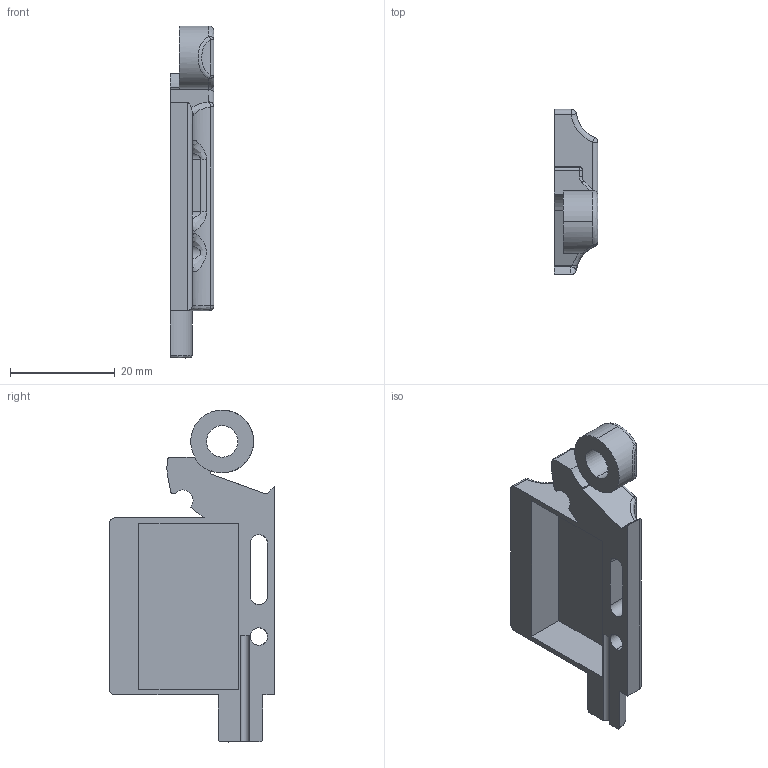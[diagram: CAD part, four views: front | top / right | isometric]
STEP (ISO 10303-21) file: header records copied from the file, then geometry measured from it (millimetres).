
FILE_DESCRIPTION (( 'STEP AP214' ), '1' );
FILE_NAME ('Imura_V3_Striker_Right.step', '2015-04-30T21:15:10', ( 'WarFairy' ), ( '' ), 'SwSTEP 2.0', 'SolidWorks 2013', '' );
FILE_SCHEMA (( 'AUTOMOTIVE_DESIGN' ));
Length unit declared in the file: millimetre
Products named in the file (1): Imura_V3_Striker_Right
Bounding box: 8.35 x 31.5 x 63.35 mm (x, y, z)
Volume: 4736.6 mm3; surface area: 4932.9 mm2
Topology: 1 solids, 1 shells, 107 faces, 271 edges, 159 vertices
Faces by surface type: cylinder 45, bspline 33, plane 25, torus 3, sphere 1
Entity records: 4877 total; most frequent: CARTESIAN_POINT 2529, ORIENTED_EDGE 530, DIRECTION 434, EDGE_CURVE 265, AXIS2_PLACEMENT_3D 161, VERTEX_POINT 159, EDGE_LOOP 112, VECTOR 112
